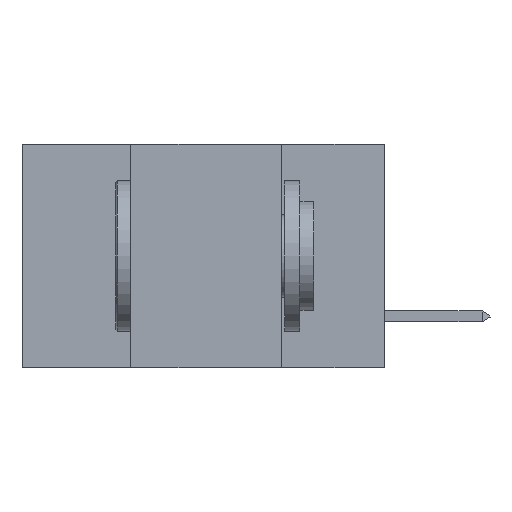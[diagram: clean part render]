
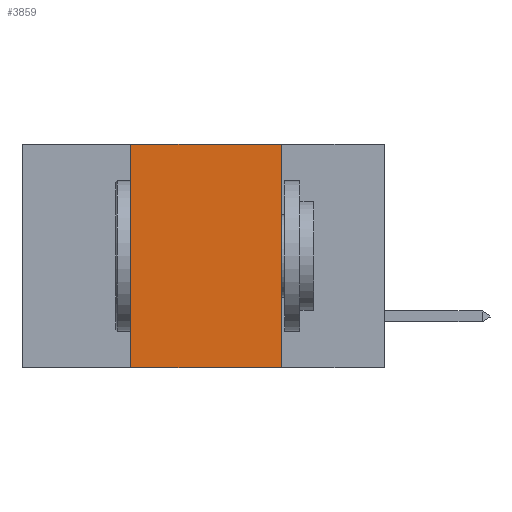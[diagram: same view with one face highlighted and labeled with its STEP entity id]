
A CAD part, left-side view. The second image highlights one B-rep face of the part: STEP entity #3859.
In plain terms, the highlighted planar face has unit normal (-1, 0, 0).
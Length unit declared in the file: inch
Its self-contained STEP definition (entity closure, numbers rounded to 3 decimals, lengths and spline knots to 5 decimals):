
#128 = VECTOR ( 'NONE', #10997, 39.37008 ) ;
#645 = DIRECTION ( 'NONE',  ( 0., 0., -1. ) ) ;
#756 = VERTEX_POINT ( 'NONE', #5873 ) ;
#773 = LINE ( 'NONE', #7084, #9060 ) ;
#912 = CARTESIAN_POINT ( 'NONE',  ( 0., 0.42, -0.37 ) ) ;
#920 = VERTEX_POINT ( 'NONE', #2268 ) ;
#1162 = ORIENTED_EDGE ( 'NONE', *, *, #13301, .T. ) ;
#1656 = ORIENTED_EDGE ( 'NONE', *, *, #7653, .F. ) ;
#1732 = VERTEX_POINT ( 'NONE', #912 ) ;
#2268 = CARTESIAN_POINT ( 'NONE',  ( 0., 0.17, -0.37 ) ) ;
#2548 = CARTESIAN_POINT ( 'NONE',  ( 0., 0.6, -0.37 ) ) ;
#2550 = CARTESIAN_POINT ( 'NONE',  ( 0., 0.17, 0. ) ) ;
#2984 = AXIS2_PLACEMENT_3D ( 'NONE', #5325, #12983, #6365 ) ;
#3050 = VECTOR ( 'NONE', #12900, 39.37008 ) ;
#3859 = ADVANCED_FACE ( 'NONE', ( #13771 ), #8479, .F. ) ;
#5325 = CARTESIAN_POINT ( 'NONE',  ( 0., 0.6, 0. ) ) ;
#5873 = CARTESIAN_POINT ( 'NONE',  ( 0., 0.42, 0. ) ) ;
#5913 = ORIENTED_EDGE ( 'NONE', *, *, #9717, .F. ) ;
#5924 = ORIENTED_EDGE ( 'NONE', *, *, #11540, .F. ) ;
#6365 = DIRECTION ( 'NONE',  ( 0., 0., -1. ) ) ;
#6814 = VECTOR ( 'NONE', #9124, 39.37008 ) ;
#7084 = CARTESIAN_POINT ( 'NONE',  ( 0., 0.17, 0. ) ) ;
#7653 = EDGE_CURVE ( 'NONE', #756, #13183, #11974, .T. ) ;
#8479 = PLANE ( 'NONE',  #2984 ) ;
#9060 = VECTOR ( 'NONE', #645, 39.37008 ) ;
#9124 = DIRECTION ( 'NONE',  ( 0., -1., 0. ) ) ;
#9717 = EDGE_CURVE ( 'NONE', #13183, #920, #773, .T. ) ;
#9728 = LINE ( 'NONE', #2548, #6814 ) ;
#9730 = CARTESIAN_POINT ( 'NONE',  ( 0., 0.42, 0. ) ) ;
#10118 = LINE ( 'NONE', #9730, #128 ) ;
#10997 = DIRECTION ( 'NONE',  ( 0., 0., 1. ) ) ;
#11540 = EDGE_CURVE ( 'NONE', #1732, #756, #10118, .T. ) ;
#11865 = CARTESIAN_POINT ( 'NONE',  ( 0., 0.6, 0. ) ) ;
#11974 = LINE ( 'NONE', #11865, #3050 ) ;
#12900 = DIRECTION ( 'NONE',  ( 0., -1., 0. ) ) ;
#12983 = DIRECTION ( 'NONE',  ( 1., 0., 0. ) ) ;
#13183 = VERTEX_POINT ( 'NONE', #2550 ) ;
#13301 = EDGE_CURVE ( 'NONE', #1732, #920, #9728, .T. ) ;
#13744 = EDGE_LOOP ( 'NONE', ( #5913, #1656, #5924, #1162 ) ) ;
#13771 = FACE_OUTER_BOUND ( 'NONE', #13744, .T. ) ;
